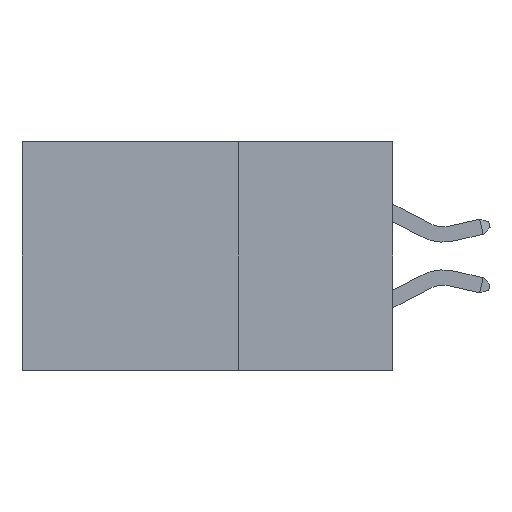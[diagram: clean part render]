
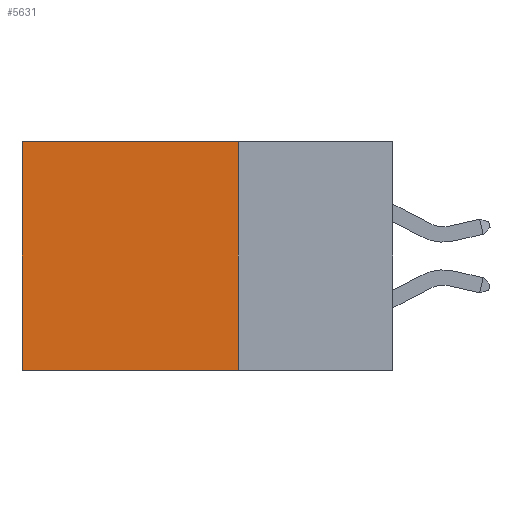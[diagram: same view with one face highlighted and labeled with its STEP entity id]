
A CAD part, left-side view. The second image highlights one B-rep face of the part: STEP entity #5631.
In plain terms, the highlighted planar face has unit normal (-1, 0, 0).
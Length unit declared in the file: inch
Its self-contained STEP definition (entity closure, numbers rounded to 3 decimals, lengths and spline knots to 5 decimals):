
#98 = VECTOR ( 'NONE', #6011, 39.37008 ) ;
#856 = VERTEX_POINT ( 'NONE', #8562 ) ;
#2008 = LINE ( 'NONE', #2393, #3873 ) ;
#2014 = ORIENTED_EDGE ( 'NONE', *, *, #9003, .F. ) ;
#2039 = ORIENTED_EDGE ( 'NONE', *, *, #9072, .F. ) ;
#2050 = LINE ( 'NONE', #4326, #4208 ) ;
#2393 = CARTESIAN_POINT ( 'NONE',  ( 0.2875, 0.6, 0. ) ) ;
#3108 = CARTESIAN_POINT ( 'NONE',  ( 0.2875, 0.25, -0.37 ) ) ;
#3321 = CARTESIAN_POINT ( 'NONE',  ( 0.2875, 0.25, 0. ) ) ;
#3334 = DIRECTION ( 'NONE',  ( 0., 0., -1. ) ) ;
#3345 = LINE ( 'NONE', #3321, #10049 ) ;
#3376 = PLANE ( 'NONE',  #9024 ) ;
#3873 = VECTOR ( 'NONE', #3334, 39.37008 ) ;
#4133 = FACE_OUTER_BOUND ( 'NONE', #8448, .T. ) ;
#4208 = VECTOR ( 'NONE', #5219, 39.37008 ) ;
#4326 = CARTESIAN_POINT ( 'NONE',  ( 0.2875, 0.25, -0.37 ) ) ;
#4357 = EDGE_CURVE ( 'NONE', #856, #6564, #2008, .T. ) ;
#4772 = VERTEX_POINT ( 'NONE', #3108 ) ;
#4779 = VERTEX_POINT ( 'NONE', #10120 ) ;
#5038 = LINE ( 'NONE', #8508, #98 ) ;
#5175 = DIRECTION ( 'NONE',  ( 0., 0., -1. ) ) ;
#5219 = DIRECTION ( 'NONE',  ( 0., 1., 0. ) ) ;
#5631 = ADVANCED_FACE ( 'NONE', ( #4133 ), #3376, .F. ) ;
#6011 = DIRECTION ( 'NONE',  ( 0., 0., -1. ) ) ;
#6564 = VERTEX_POINT ( 'NONE', #8953 ) ;
#7579 = ORIENTED_EDGE ( 'NONE', *, *, #4357, .T. ) ;
#8448 = EDGE_LOOP ( 'NONE', ( #7579, #2039, #2014, #8668 ) ) ;
#8508 = CARTESIAN_POINT ( 'NONE',  ( 0.2875, 0.25, 0. ) ) ;
#8562 = CARTESIAN_POINT ( 'NONE',  ( 0.2875, 0.6, 0. ) ) ;
#8668 = ORIENTED_EDGE ( 'NONE', *, *, #9654, .T. ) ;
#8953 = CARTESIAN_POINT ( 'NONE',  ( 0.2875, 0.6, -0.37 ) ) ;
#9003 = EDGE_CURVE ( 'NONE', #4779, #4772, #5038, .T. ) ;
#9024 = AXIS2_PLACEMENT_3D ( 'NONE', #9460, #10384, #5175 ) ;
#9072 = EDGE_CURVE ( 'NONE', #4772, #6564, #2050, .T. ) ;
#9410 = DIRECTION ( 'NONE',  ( 0., 1., 0. ) ) ;
#9460 = CARTESIAN_POINT ( 'NONE',  ( 0.2875, 0.25, 0. ) ) ;
#9654 = EDGE_CURVE ( 'NONE', #4779, #856, #3345, .T. ) ;
#10049 = VECTOR ( 'NONE', #9410, 39.37008 ) ;
#10120 = CARTESIAN_POINT ( 'NONE',  ( 0.2875, 0.25, 0. ) ) ;
#10384 = DIRECTION ( 'NONE',  ( 1., 0., 0. ) ) ;
